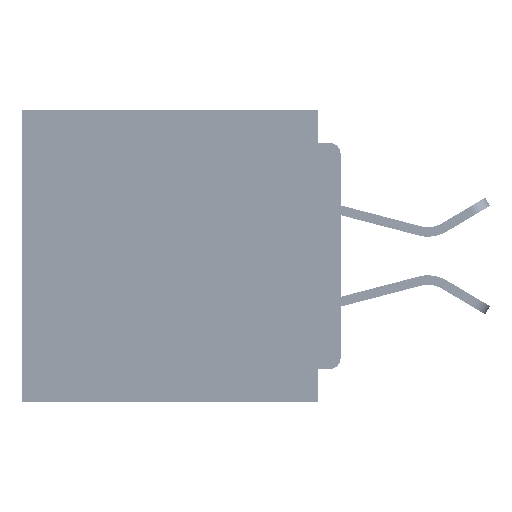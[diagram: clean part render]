
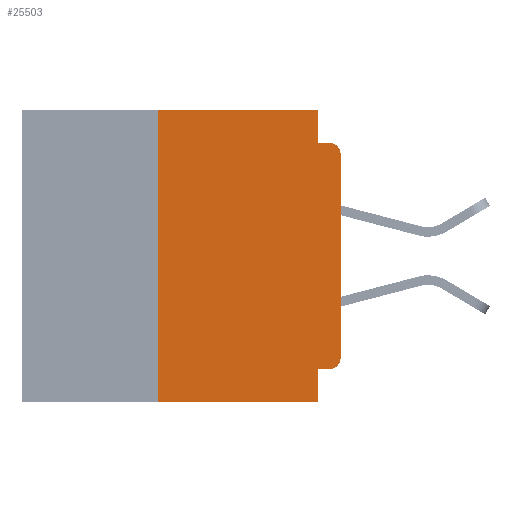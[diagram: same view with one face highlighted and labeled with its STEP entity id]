
A CAD part, left-side view. The second image highlights one B-rep face of the part: STEP entity #25503.
In plain terms, the highlighted planar face has unit normal (-1, 0, 0).
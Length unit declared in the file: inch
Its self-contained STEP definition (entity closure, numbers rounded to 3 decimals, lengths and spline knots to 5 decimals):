
#1511 = CARTESIAN_POINT ( 'NONE',  ( 0., 0.031, -0.4 ) ) ;
#1752 = ORIENTED_EDGE ( 'NONE', *, *, #32264, .F. ) ;
#1780 = FACE_OUTER_BOUND ( 'NONE', #56480, .T. ) ;
#2839 = CIRCLE ( 'NONE', #17079, 0.015 ) ;
#3516 = VERTEX_POINT ( 'NONE', #24643 ) ;
#4132 = DIRECTION ( 'NONE',  ( -1., 0., 0. ) ) ;
#5724 = ORIENTED_EDGE ( 'NONE', *, *, #12063, .F. ) ;
#8040 = LINE ( 'NONE', #42752, #58463 ) ;
#8296 = EDGE_CURVE ( 'NONE', #3516, #13674, #14944, .T. ) ;
#8549 = DIRECTION ( 'NONE',  ( 0., 0., 1. ) ) ;
#8844 = CARTESIAN_POINT ( 'NONE',  ( 0., 0., -0.045 ) ) ;
#9293 = DIRECTION ( 'NONE',  ( 0., 0., -1. ) ) ;
#9369 = CARTESIAN_POINT ( 'NONE',  ( 0., 0.031, -0.045 ) ) ;
#9569 = DIRECTION ( 'NONE',  ( -1., 0., 0. ) ) ;
#10529 = DIRECTION ( 'NONE',  ( 0., 0., -1. ) ) ;
#11819 = EDGE_CURVE ( 'NONE', #39175, #13674, #13803, .T. ) ;
#12063 = EDGE_CURVE ( 'NONE', #34565, #40561, #27587, .T. ) ;
#12247 = VECTOR ( 'NONE', #43080, 39.37008 ) ;
#12465 = EDGE_CURVE ( 'NONE', #57384, #3516, #29055, .T. ) ;
#13674 = VERTEX_POINT ( 'NONE', #35932 ) ;
#13803 = LINE ( 'NONE', #8844, #12247 ) ;
#14540 = CARTESIAN_POINT ( 'NONE',  ( 0., 0.015, -0.355 ) ) ;
#14944 = CIRCLE ( 'NONE', #52135, 0.015 ) ;
#16043 = EDGE_CURVE ( 'NONE', #27151, #40561, #8040, .T. ) ;
#16791 = EDGE_CURVE ( 'NONE', #35582, #39175, #54550, .T. ) ;
#16844 = ORIENTED_EDGE ( 'NONE', *, *, #16043, .T. ) ;
#17079 = AXIS2_PLACEMENT_3D ( 'NONE', #38911, #9569, #43804 ) ;
#18284 = DIRECTION ( 'NONE',  ( 0., -1., 0. ) ) ;
#18398 = DIRECTION ( 'NONE',  ( 0., -1., 0. ) ) ;
#19219 = CARTESIAN_POINT ( 'NONE',  ( 0., 0.031, -0.355 ) ) ;
#19893 = CARTESIAN_POINT ( 'NONE',  ( 0., 0.25, 0. ) ) ;
#24015 = ORIENTED_EDGE ( 'NONE', *, *, #61133, .F. ) ;
#24643 = CARTESIAN_POINT ( 'NONE',  ( 0., 0., -0.06 ) ) ;
#24690 = DIRECTION ( 'NONE',  ( 0., 0., -1. ) ) ;
#24806 = ORIENTED_EDGE ( 'NONE', *, *, #12465, .T. ) ;
#25503 = ADVANCED_FACE ( 'NONE', ( #1780 ), #34317, .F. ) ;
#26016 = VECTOR ( 'NONE', #10529, 39.37008 ) ;
#26712 = DIRECTION ( 'NONE',  ( 0., 0., 1. ) ) ;
#27151 = VERTEX_POINT ( 'NONE', #50674 ) ;
#27587 = LINE ( 'NONE', #30271, #26016 ) ;
#27819 = ORIENTED_EDGE ( 'NONE', *, *, #56403, .F. ) ;
#28019 = VECTOR ( 'NONE', #8549, 39.37008 ) ;
#28147 = CARTESIAN_POINT ( 'NONE',  ( 0., 0.437, 0. ) ) ;
#29055 = LINE ( 'NONE', #38380, #53403 ) ;
#30271 = CARTESIAN_POINT ( 'NONE',  ( 0., 0.031, -0.4 ) ) ;
#32264 = EDGE_CURVE ( 'NONE', #27151, #42467, #53895, .T. ) ;
#33443 = CARTESIAN_POINT ( 'NONE',  ( 0., 0.015, -0.06 ) ) ;
#34317 = PLANE ( 'NONE',  #60258 ) ;
#34533 = LINE ( 'NONE', #57060, #55813 ) ;
#34565 = VERTEX_POINT ( 'NONE', #19219 ) ;
#35582 = VERTEX_POINT ( 'NONE', #41745 ) ;
#35932 = CARTESIAN_POINT ( 'NONE',  ( 0., 0.015, -0.045 ) ) ;
#38327 = DIRECTION ( 'NONE',  ( 0., 0., -1. ) ) ;
#38380 = CARTESIAN_POINT ( 'NONE',  ( 0., 0., 0. ) ) ;
#38911 = CARTESIAN_POINT ( 'NONE',  ( 0., 0.015, -0.34 ) ) ;
#39175 = VERTEX_POINT ( 'NONE', #9369 ) ;
#40561 = VERTEX_POINT ( 'NONE', #1511 ) ;
#41745 = CARTESIAN_POINT ( 'NONE',  ( 0., 0.031, 0. ) ) ;
#42467 = VERTEX_POINT ( 'NONE', #19893 ) ;
#42752 = CARTESIAN_POINT ( 'NONE',  ( 0., 0.437, -0.4 ) ) ;
#43080 = DIRECTION ( 'NONE',  ( 0., -1., 0. ) ) ;
#43163 = VECTOR ( 'NONE', #9293, 39.37008 ) ;
#43514 = CARTESIAN_POINT ( 'NONE',  ( 0., 0.031, 0. ) ) ;
#43804 = DIRECTION ( 'NONE',  ( 0., 0., -1. ) ) ;
#43900 = CARTESIAN_POINT ( 'NONE',  ( 0., 0.437, 0. ) ) ;
#45553 = ORIENTED_EDGE ( 'NONE', *, *, #11819, .F. ) ;
#47153 = LINE ( 'NONE', #28147, #58559 ) ;
#47981 = ORIENTED_EDGE ( 'NONE', *, *, #63146, .T. ) ;
#50674 = CARTESIAN_POINT ( 'NONE',  ( 0., 0.25, -0.4 ) ) ;
#52135 = AXIS2_PLACEMENT_3D ( 'NONE', #33443, #4132, #38327 ) ;
#53385 = VERTEX_POINT ( 'NONE', #14540 ) ;
#53403 = VECTOR ( 'NONE', #26712, 39.37008 ) ;
#53853 = DIRECTION ( 'NONE',  ( 1., 0., 0. ) ) ;
#53895 = LINE ( 'NONE', #62079, #28019 ) ;
#54550 = LINE ( 'NONE', #43514, #43163 ) ;
#55813 = VECTOR ( 'NONE', #61934, 39.37008 ) ;
#56403 = EDGE_CURVE ( 'NONE', #42467, #35582, #47153, .T. ) ;
#56480 = EDGE_LOOP ( 'NONE', ( #24806, #62235, #45553, #61095, #27819, #1752, #16844, #5724, #24015, #47981 ) ) ;
#57060 = CARTESIAN_POINT ( 'NONE',  ( 0., 0., -0.355 ) ) ;
#57384 = VERTEX_POINT ( 'NONE', #59318 ) ;
#58463 = VECTOR ( 'NONE', #18398, 39.37008 ) ;
#58559 = VECTOR ( 'NONE', #18284, 39.37008 ) ;
#59318 = CARTESIAN_POINT ( 'NONE',  ( 0., 0., -0.34 ) ) ;
#60258 = AXIS2_PLACEMENT_3D ( 'NONE', #43900, #53853, #24690 ) ;
#61095 = ORIENTED_EDGE ( 'NONE', *, *, #16791, .F. ) ;
#61133 = EDGE_CURVE ( 'NONE', #53385, #34565, #34533, .T. ) ;
#61934 = DIRECTION ( 'NONE',  ( 0., 1., 0. ) ) ;
#62079 = CARTESIAN_POINT ( 'NONE',  ( 0., 0.25, -0.4 ) ) ;
#62235 = ORIENTED_EDGE ( 'NONE', *, *, #8296, .T. ) ;
#63146 = EDGE_CURVE ( 'NONE', #53385, #57384, #2839, .T. ) ;
